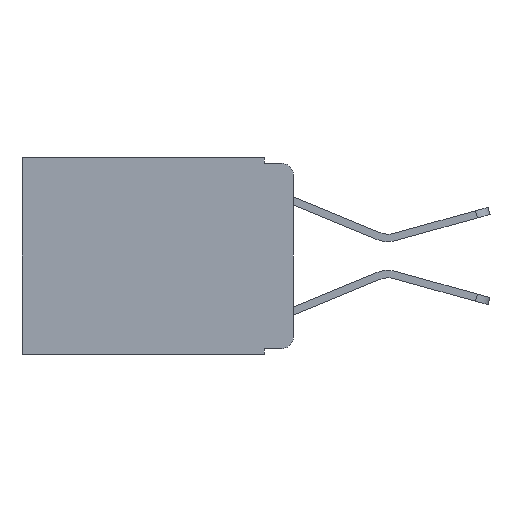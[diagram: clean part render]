
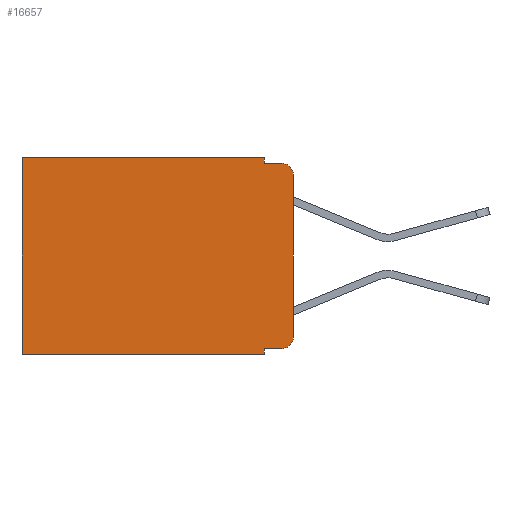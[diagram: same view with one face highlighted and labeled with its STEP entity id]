
A CAD part, left-side view. The second image highlights one B-rep face of the part: STEP entity #16657.
In plain terms, the highlighted planar face has unit normal (-1, 0, 0).
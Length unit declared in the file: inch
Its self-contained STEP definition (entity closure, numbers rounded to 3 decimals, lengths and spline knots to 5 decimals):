
#118 = VERTEX_POINT ( 'NONE', #19334 ) ;
#180 = VECTOR ( 'NONE', #5974, 39.37008 ) ;
#515 = EDGE_LOOP ( 'NONE', ( #15134, #17569, #1798, #13018, #1491, #17877, #13640, #4306, #17285, #19959 ) ) ;
#615 = EDGE_CURVE ( 'NONE', #4137, #23085, #21867, .T. ) ;
#814 = LINE ( 'NONE', #4779, #180 ) ;
#956 = CARTESIAN_POINT ( 'NONE',  ( 0.298, 0.051, 0. ) ) ;
#1067 = EDGE_CURVE ( 'NONE', #18115, #22670, #6951, .T. ) ;
#1270 = VERTEX_POINT ( 'NONE', #9562 ) ;
#1491 = ORIENTED_EDGE ( 'NONE', *, *, #3077, .T. ) ;
#1526 = LINE ( 'NONE', #15572, #21767 ) ;
#1798 = ORIENTED_EDGE ( 'NONE', *, *, #1067, .F. ) ;
#2177 = CIRCLE ( 'NONE', #16939, 0.02 ) ;
#2239 = VECTOR ( 'NONE', #20520, 39.37008 ) ;
#2415 = EDGE_CURVE ( 'NONE', #19472, #18115, #25061, .T. ) ;
#3077 = EDGE_CURVE ( 'NONE', #19472, #7520, #16439, .T. ) ;
#3217 = EDGE_CURVE ( 'NONE', #118, #22670, #2177, .T. ) ;
#3758 = EDGE_CURVE ( 'NONE', #7520, #23085, #1526, .T. ) ;
#3980 = CARTESIAN_POINT ( 'NONE',  ( 0.298, 0., -0.343 ) ) ;
#4067 = CARTESIAN_POINT ( 'NONE',  ( 0.298, 0., 0. ) ) ;
#4137 = VERTEX_POINT ( 'NONE', #10913 ) ;
#4306 = ORIENTED_EDGE ( 'NONE', *, *, #5134, .F. ) ;
#4515 = CARTESIAN_POINT ( 'NONE',  ( 0.298, 0., 0. ) ) ;
#4779 = CARTESIAN_POINT ( 'NONE',  ( 0.298, 0.051, 0. ) ) ;
#4844 = DIRECTION ( 'NONE',  ( 0., -1., 0. ) ) ;
#5134 = EDGE_CURVE ( 'NONE', #10683, #4137, #814, .T. ) ;
#5973 = VECTOR ( 'NONE', #15539, 39.37008 ) ;
#5974 = DIRECTION ( 'NONE',  ( 0., 0., -1. ) ) ;
#6104 = PLANE ( 'NONE',  #20621 ) ;
#6356 = VECTOR ( 'NONE', #24963, 39.37008 ) ;
#6871 = CARTESIAN_POINT ( 'NONE',  ( 0.298, 0.051, -0.333 ) ) ;
#6951 = LINE ( 'NONE', #20854, #2239 ) ;
#7209 = DIRECTION ( 'NONE',  ( -1., 0., 0. ) ) ;
#7226 = FACE_OUTER_BOUND ( 'NONE', #515, .T. ) ;
#7330 = CARTESIAN_POINT ( 'NONE',  ( 0.298, 0.473, -0.343 ) ) ;
#7520 = VERTEX_POINT ( 'NONE', #17676 ) ;
#7792 = EDGE_CURVE ( 'NONE', #10683, #1270, #11195, .T. ) ;
#8881 = DIRECTION ( 'NONE',  ( 0., 0., -1. ) ) ;
#9127 = EDGE_CURVE ( 'NONE', #1270, #13937, #17821, .T. ) ;
#9508 = DIRECTION ( 'NONE',  ( 0., 0., -1. ) ) ;
#9562 = CARTESIAN_POINT ( 'NONE',  ( 0.298, 0.02, -0.333 ) ) ;
#9624 = DIRECTION ( 'NONE',  ( -1., 0., 0. ) ) ;
#10082 = DIRECTION ( 'NONE',  ( 0., 0., -1. ) ) ;
#10683 = VERTEX_POINT ( 'NONE', #20283 ) ;
#10913 = CARTESIAN_POINT ( 'NONE',  ( 0.298, 0.051, -0.343 ) ) ;
#11195 = LINE ( 'NONE', #6871, #15186 ) ;
#11610 = AXIS2_PLACEMENT_3D ( 'NONE', #18932, #7209, #20831 ) ;
#13018 = ORIENTED_EDGE ( 'NONE', *, *, #2415, .F. ) ;
#13640 = ORIENTED_EDGE ( 'NONE', *, *, #615, .F. ) ;
#13937 = VERTEX_POINT ( 'NONE', #24620 ) ;
#14486 = VECTOR ( 'NONE', #20247, 39.37008 ) ;
#15134 = ORIENTED_EDGE ( 'NONE', *, *, #19354, .F. ) ;
#15186 = VECTOR ( 'NONE', #4844, 39.37008 ) ;
#15539 = DIRECTION ( 'NONE',  ( 0., 1., 0. ) ) ;
#15572 = CARTESIAN_POINT ( 'NONE',  ( 0.298, 0.473, 0. ) ) ;
#15856 = CARTESIAN_POINT ( 'NONE',  ( 0.298, 0.02, -0.03 ) ) ;
#16420 = DIRECTION ( 'NONE',  ( 0., 0., -1. ) ) ;
#16439 = LINE ( 'NONE', #4515, #5973 ) ;
#16657 = ADVANCED_FACE ( 'NONE', ( #7226 ), #6104, .F. ) ;
#16939 = AXIS2_PLACEMENT_3D ( 'NONE', #15856, #9624, #9508 ) ;
#17285 = ORIENTED_EDGE ( 'NONE', *, *, #7792, .T. ) ;
#17569 = ORIENTED_EDGE ( 'NONE', *, *, #3217, .T. ) ;
#17676 = CARTESIAN_POINT ( 'NONE',  ( 0.298, 0.473, 0. ) ) ;
#17810 = CARTESIAN_POINT ( 'NONE',  ( 0.298, 0.02, -0.01 ) ) ;
#17821 = CIRCLE ( 'NONE', #11610, 0.02 ) ;
#17877 = ORIENTED_EDGE ( 'NONE', *, *, #3758, .T. ) ;
#18115 = VERTEX_POINT ( 'NONE', #18219 ) ;
#18219 = CARTESIAN_POINT ( 'NONE',  ( 0.298, 0.051, -0.01 ) ) ;
#18331 = CARTESIAN_POINT ( 'NONE',  ( 0.298, 0., 0. ) ) ;
#18742 = CARTESIAN_POINT ( 'NONE',  ( 0.298, 0.051, 0. ) ) ;
#18932 = CARTESIAN_POINT ( 'NONE',  ( 0.298, 0.02, -0.313 ) ) ;
#19334 = CARTESIAN_POINT ( 'NONE',  ( 0.298, 0., -0.03 ) ) ;
#19354 = EDGE_CURVE ( 'NONE', #118, #13937, #19610, .T. ) ;
#19472 = VERTEX_POINT ( 'NONE', #18742 ) ;
#19610 = LINE ( 'NONE', #18331, #14486 ) ;
#19959 = ORIENTED_EDGE ( 'NONE', *, *, #9127, .T. ) ;
#20055 = VECTOR ( 'NONE', #8881, 39.37008 ) ;
#20247 = DIRECTION ( 'NONE',  ( 0., 0., -1. ) ) ;
#20283 = CARTESIAN_POINT ( 'NONE',  ( 0.298, 0.051, -0.333 ) ) ;
#20520 = DIRECTION ( 'NONE',  ( 0., -1., 0. ) ) ;
#20621 = AXIS2_PLACEMENT_3D ( 'NONE', #4067, #21668, #10082 ) ;
#20831 = DIRECTION ( 'NONE',  ( 0., 0., -1. ) ) ;
#20854 = CARTESIAN_POINT ( 'NONE',  ( 0.298, 0.051, -0.01 ) ) ;
#21668 = DIRECTION ( 'NONE',  ( 1., 0., 0. ) ) ;
#21767 = VECTOR ( 'NONE', #16420, 39.37008 ) ;
#21867 = LINE ( 'NONE', #3980, #6356 ) ;
#22670 = VERTEX_POINT ( 'NONE', #17810 ) ;
#23085 = VERTEX_POINT ( 'NONE', #7330 ) ;
#24620 = CARTESIAN_POINT ( 'NONE',  ( 0.298, 0., -0.313 ) ) ;
#24963 = DIRECTION ( 'NONE',  ( 0., 1., 0. ) ) ;
#25061 = LINE ( 'NONE', #956, #20055 ) ;
